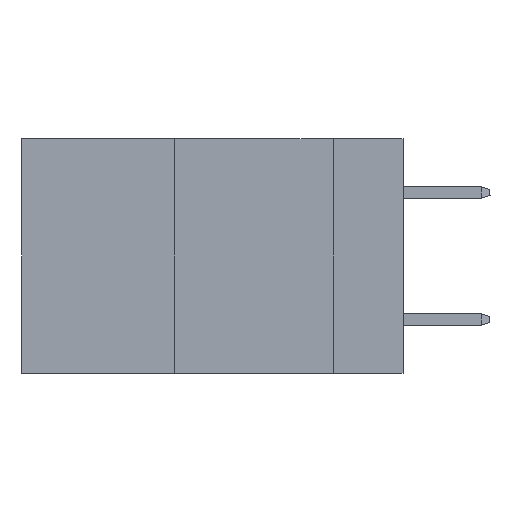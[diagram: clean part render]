
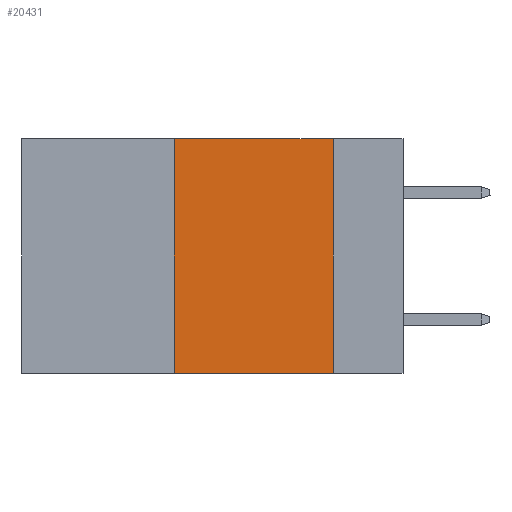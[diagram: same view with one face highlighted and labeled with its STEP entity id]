
A CAD part, left-side view. The second image highlights one B-rep face of the part: STEP entity #20431.
In plain terms, the highlighted planar face has unit normal (-1, 0, 0).
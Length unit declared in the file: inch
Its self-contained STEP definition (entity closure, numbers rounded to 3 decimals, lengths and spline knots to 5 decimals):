
#255 = CARTESIAN_POINT ( 'NONE',  ( 0., 0.6, 0. ) ) ;
#1735 = DIRECTION ( 'NONE',  ( 0., -1., 0. ) ) ;
#2269 = PLANE ( 'NONE',  #17424 ) ;
#3163 = EDGE_CURVE ( 'NONE', #12505, #12991, #14729, .T. ) ;
#3529 = EDGE_CURVE ( 'NONE', #12505, #19402, #10292, .T. ) ;
#4208 = DIRECTION ( 'NONE',  ( 0., 0., -1. ) ) ;
#5590 = DIRECTION ( 'NONE',  ( 0., -1., 0. ) ) ;
#5841 = VECTOR ( 'NONE', #5590, 39.37008 ) ;
#7300 = LINE ( 'NONE', #19156, #17279 ) ;
#7319 = DIRECTION ( 'NONE',  ( 0., 0., -1. ) ) ;
#7360 = LINE ( 'NONE', #255, #5841 ) ;
#7741 = VECTOR ( 'NONE', #9772, 39.37008 ) ;
#8971 = CARTESIAN_POINT ( 'NONE',  ( 0., 0.6, 0. ) ) ;
#9772 = DIRECTION ( 'NONE',  ( 0., 0., 1. ) ) ;
#10292 = LINE ( 'NONE', #16648, #11204 ) ;
#11204 = VECTOR ( 'NONE', #1735, 39.37008 ) ;
#12505 = VERTEX_POINT ( 'NONE', #14932 ) ;
#12592 = ORIENTED_EDGE ( 'NONE', *, *, #3529, .T. ) ;
#12991 = VERTEX_POINT ( 'NONE', #19266 ) ;
#13040 = CARTESIAN_POINT ( 'NONE',  ( 0., 0.11, -0.37 ) ) ;
#13574 = VERTEX_POINT ( 'NONE', #20169 ) ;
#13619 = EDGE_LOOP ( 'NONE', ( #13878, #21269, #14791, #12592 ) ) ;
#13878 = ORIENTED_EDGE ( 'NONE', *, *, #13925, .F. ) ;
#13925 = EDGE_CURVE ( 'NONE', #13574, #19402, #7300, .T. ) ;
#14657 = EDGE_CURVE ( 'NONE', #12991, #13574, #7360, .T. ) ;
#14729 = LINE ( 'NONE', #19851, #7741 ) ;
#14791 = ORIENTED_EDGE ( 'NONE', *, *, #3163, .F. ) ;
#14932 = CARTESIAN_POINT ( 'NONE',  ( 0., 0.36, -0.37 ) ) ;
#15530 = DIRECTION ( 'NONE',  ( 1., 0., 0. ) ) ;
#16648 = CARTESIAN_POINT ( 'NONE',  ( 0., 0.6, -0.37 ) ) ;
#17196 = FACE_OUTER_BOUND ( 'NONE', #13619, .T. ) ;
#17279 = VECTOR ( 'NONE', #4208, 39.37008 ) ;
#17424 = AXIS2_PLACEMENT_3D ( 'NONE', #8971, #15530, #7319 ) ;
#19156 = CARTESIAN_POINT ( 'NONE',  ( 0., 0.11, 0. ) ) ;
#19266 = CARTESIAN_POINT ( 'NONE',  ( 0., 0.36, 0. ) ) ;
#19402 = VERTEX_POINT ( 'NONE', #13040 ) ;
#19851 = CARTESIAN_POINT ( 'NONE',  ( 0., 0.36, 0. ) ) ;
#20169 = CARTESIAN_POINT ( 'NONE',  ( 0., 0.11, 0. ) ) ;
#20431 = ADVANCED_FACE ( 'NONE', ( #17196 ), #2269, .F. ) ;
#21269 = ORIENTED_EDGE ( 'NONE', *, *, #14657, .F. ) ;
